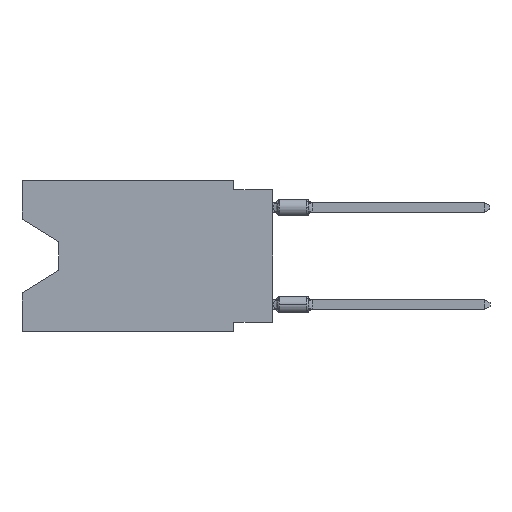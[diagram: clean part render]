
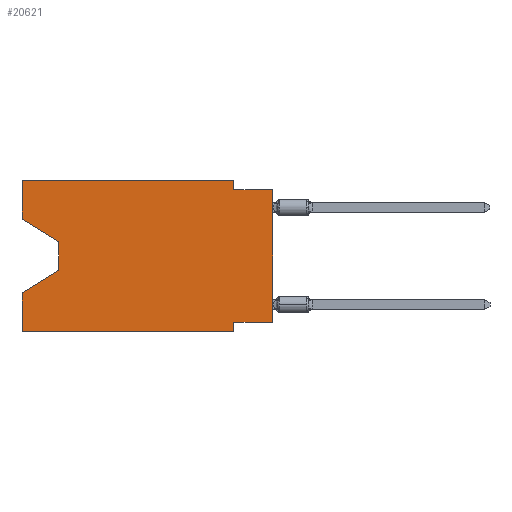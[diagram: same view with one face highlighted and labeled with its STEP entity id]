
A CAD part, left-side view. The second image highlights one B-rep face of the part: STEP entity #20621.
In plain terms, the highlighted planar face has unit normal (-1, 0, 0).
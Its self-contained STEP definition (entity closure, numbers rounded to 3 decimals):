
#525 = EDGE_CURVE ( 'NONE', #10009, #16439, #11002, .T. ) ;
#1297 = EDGE_CURVE ( 'NONE', #3603, #21370, #16204, .T. ) ;
#1332 = VECTOR ( 'NONE', #16612, 1000. ) ;
#1543 = VERTEX_POINT ( 'NONE', #10751 ) ;
#2050 = CARTESIAN_POINT ( 'NONE',  ( 0., 16.383, -9.906 ) ) ;
#2188 = VECTOR ( 'NONE', #19710, 1000. ) ;
#2782 = DIRECTION ( 'NONE',  ( 0., -0.855, -0.519 ) ) ;
#3603 = VERTEX_POINT ( 'NONE', #8439 ) ;
#3914 = VECTOR ( 'NONE', #22411, 1000. ) ;
#4243 = ORIENTED_EDGE ( 'NONE', *, *, #24128, .F. ) ;
#4929 = VECTOR ( 'NONE', #7525, 1000. ) ;
#5431 = FACE_OUTER_BOUND ( 'NONE', #23763, .T. ) ;
#5456 = CARTESIAN_POINT ( 'NONE',  ( 0., 0., -0.635 ) ) ;
#6255 = VERTEX_POINT ( 'NONE', #23429 ) ;
#6332 = CARTESIAN_POINT ( 'NONE',  ( 0., 16.383, -2.546 ) ) ;
#6381 = VECTOR ( 'NONE', #23459, 1000. ) ;
#6884 = CARTESIAN_POINT ( 'NONE',  ( 0., 0., 0. ) ) ;
#7053 = LINE ( 'NONE', #5456, #15903 ) ;
#7405 = ORIENTED_EDGE ( 'NONE', *, *, #1297, .F. ) ;
#7525 = DIRECTION ( 'NONE',  ( 0., 0., 1. ) ) ;
#7762 = CARTESIAN_POINT ( 'NONE',  ( 0., 16.383, 0. ) ) ;
#7830 = EDGE_CURVE ( 'NONE', #15887, #10565, #11643, .T. ) ;
#8192 = ORIENTED_EDGE ( 'NONE', *, *, #17549, .T. ) ;
#8243 = VERTEX_POINT ( 'NONE', #13346 ) ;
#8361 = VECTOR ( 'NONE', #17067, 1000. ) ;
#8439 = CARTESIAN_POINT ( 'NONE',  ( 0., 16.383, -2.546 ) ) ;
#8836 = VERTEX_POINT ( 'NONE', #11030 ) ;
#9110 = CARTESIAN_POINT ( 'NONE',  ( 0., 2.54, -0.635 ) ) ;
#9308 = AXIS2_PLACEMENT_3D ( 'NONE', #12619, #16547, #11146 ) ;
#9345 = CARTESIAN_POINT ( 'NONE',  ( 0., 16.383, 0. ) ) ;
#10009 = VERTEX_POINT ( 'NONE', #14046 ) ;
#10418 = VERTEX_POINT ( 'NONE', #19398 ) ;
#10453 = CARTESIAN_POINT ( 'NONE',  ( 0., 16.383, 0. ) ) ;
#10507 = ORIENTED_EDGE ( 'NONE', *, *, #13955, .F. ) ;
#10565 = VERTEX_POINT ( 'NONE', #21588 ) ;
#10690 = ORIENTED_EDGE ( 'NONE', *, *, #19600, .T. ) ;
#10751 = CARTESIAN_POINT ( 'NONE',  ( 0., 0., -9.271 ) ) ;
#11002 = LINE ( 'NONE', #18611, #3914 ) ;
#11030 = CARTESIAN_POINT ( 'NONE',  ( 0., 2.54, -9.271 ) ) ;
#11062 = ORIENTED_EDGE ( 'NONE', *, *, #525, .F. ) ;
#11146 = DIRECTION ( 'NONE',  ( 0., 0., -1. ) ) ;
#11643 = LINE ( 'NONE', #13493, #12915 ) ;
#12375 = VECTOR ( 'NONE', #22669, 1000. ) ;
#12619 = CARTESIAN_POINT ( 'NONE',  ( 0., 16.383, 0. ) ) ;
#12654 = EDGE_CURVE ( 'NONE', #1543, #8836, #14671, .T. ) ;
#12915 = VECTOR ( 'NONE', #19106, 1000. ) ;
#13346 = CARTESIAN_POINT ( 'NONE',  ( 0., 0., -0.635 ) ) ;
#13493 = CARTESIAN_POINT ( 'NONE',  ( 0., 13.97, -4.013 ) ) ;
#13955 = EDGE_CURVE ( 'NONE', #21370, #10009, #15983, .T. ) ;
#14046 = CARTESIAN_POINT ( 'NONE',  ( 0., 2.54, 0. ) ) ;
#14652 = CARTESIAN_POINT ( 'NONE',  ( 0., 16.383, 0. ) ) ;
#14671 = LINE ( 'NONE', #22140, #21136 ) ;
#15202 = CARTESIAN_POINT ( 'NONE',  ( 0., 13.97, -5.893 ) ) ;
#15887 = VERTEX_POINT ( 'NONE', #17632 ) ;
#15903 = VECTOR ( 'NONE', #18768, 1000. ) ;
#15924 = CARTESIAN_POINT ( 'NONE',  ( 0., 2.54, -9.906 ) ) ;
#15983 = LINE ( 'NONE', #10453, #6381 ) ;
#16058 = EDGE_CURVE ( 'NONE', #8836, #6255, #18569, .T. ) ;
#16204 = LINE ( 'NONE', #7762, #21090 ) ;
#16439 = VERTEX_POINT ( 'NONE', #9110 ) ;
#16530 = EDGE_CURVE ( 'NONE', #21935, #6255, #18776, .T. ) ;
#16547 = DIRECTION ( 'NONE',  ( 1., 0., 0. ) ) ;
#16612 = DIRECTION ( 'NONE',  ( 0., 0., -1. ) ) ;
#16691 = LINE ( 'NONE', #9345, #4929 ) ;
#16945 = CARTESIAN_POINT ( 'NONE',  ( 0., 16.383, -9.906 ) ) ;
#17067 = DIRECTION ( 'NONE',  ( 0., -1., 0. ) ) ;
#17396 = ORIENTED_EDGE ( 'NONE', *, *, #16058, .F. ) ;
#17428 = LINE ( 'NONE', #6332, #21346 ) ;
#17539 = ORIENTED_EDGE ( 'NONE', *, *, #7830, .T. ) ;
#17549 = EDGE_CURVE ( 'NONE', #1543, #8243, #23532, .T. ) ;
#17632 = CARTESIAN_POINT ( 'NONE',  ( 0., 13.97, -4.013 ) ) ;
#17788 = ORIENTED_EDGE ( 'NONE', *, *, #19020, .F. ) ;
#18497 = PLANE ( 'NONE',  #9308 ) ;
#18569 = LINE ( 'NONE', #15924, #1332 ) ;
#18611 = CARTESIAN_POINT ( 'NONE',  ( 0., 2.54, 0. ) ) ;
#18768 = DIRECTION ( 'NONE',  ( 0., -1., 0. ) ) ;
#18776 = LINE ( 'NONE', #2050, #8361 ) ;
#19020 = EDGE_CURVE ( 'NONE', #16439, #8243, #7053, .T. ) ;
#19106 = DIRECTION ( 'NONE',  ( 0., 0., -1. ) ) ;
#19398 = CARTESIAN_POINT ( 'NONE',  ( 0., 16.383, -7.36 ) ) ;
#19600 = EDGE_CURVE ( 'NONE', #10565, #10418, #20694, .T. ) ;
#19710 = DIRECTION ( 'NONE',  ( 0., 0., 1. ) ) ;
#20286 = DIRECTION ( 'NONE',  ( 0., 1., 0. ) ) ;
#20621 = ADVANCED_FACE ( 'NONE', ( #5431 ), #18497, .F. ) ;
#20694 = LINE ( 'NONE', #15202, #12375 ) ;
#20958 = DIRECTION ( 'NONE',  ( 0., 0., 1. ) ) ;
#21090 = VECTOR ( 'NONE', #20958, 1000. ) ;
#21136 = VECTOR ( 'NONE', #20286, 1000. ) ;
#21346 = VECTOR ( 'NONE', #2782, 1000. ) ;
#21370 = VERTEX_POINT ( 'NONE', #14652 ) ;
#21588 = CARTESIAN_POINT ( 'NONE',  ( 0., 13.97, -5.893 ) ) ;
#21935 = VERTEX_POINT ( 'NONE', #16945 ) ;
#22052 = EDGE_CURVE ( 'NONE', #3603, #15887, #17428, .T. ) ;
#22140 = CARTESIAN_POINT ( 'NONE',  ( 0., 0., -9.271 ) ) ;
#22411 = DIRECTION ( 'NONE',  ( 0., 0., -1. ) ) ;
#22565 = ORIENTED_EDGE ( 'NONE', *, *, #16530, .T. ) ;
#22669 = DIRECTION ( 'NONE',  ( 0., 0.855, -0.519 ) ) ;
#22816 = ORIENTED_EDGE ( 'NONE', *, *, #22052, .T. ) ;
#23429 = CARTESIAN_POINT ( 'NONE',  ( 0., 2.54, -9.906 ) ) ;
#23459 = DIRECTION ( 'NONE',  ( 0., -1., 0. ) ) ;
#23532 = LINE ( 'NONE', #6884, #2188 ) ;
#23763 = EDGE_LOOP ( 'NONE', ( #22816, #17539, #10690, #4243, #22565, #17396, #23918, #8192, #17788, #11062, #10507, #7405 ) ) ;
#23918 = ORIENTED_EDGE ( 'NONE', *, *, #12654, .F. ) ;
#24128 = EDGE_CURVE ( 'NONE', #21935, #10418, #16691, .T. ) ;
